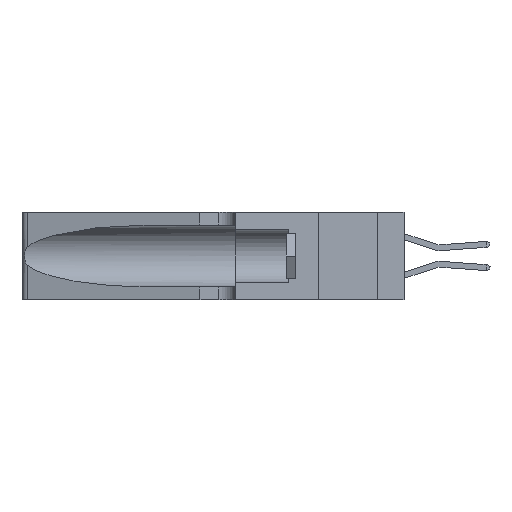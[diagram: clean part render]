
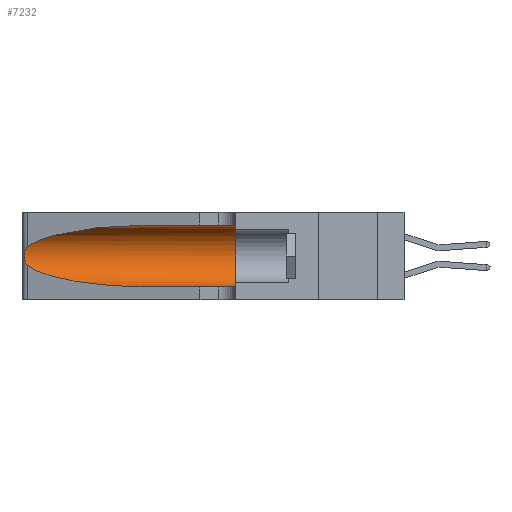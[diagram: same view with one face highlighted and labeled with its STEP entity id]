
A CAD part, left-side view. The second image highlights one B-rep face of the part: STEP entity #7232.
In plain terms, the highlighted cylindrical face has radius 3.308 mm (diameter 6.617 mm), a partial arc.
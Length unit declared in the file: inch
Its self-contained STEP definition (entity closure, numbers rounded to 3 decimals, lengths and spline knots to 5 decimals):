
#592 = FACE_OUTER_BOUND ( 'NONE', #15677, .T. ) ;
#1130 = DIRECTION ( 'NONE',  ( 0., 0., 1. ) ) ;
#1370 = VERTEX_POINT ( 'NONE', #33867 ) ;
#1551 = CARTESIAN_POINT ( 'NONE',  ( 0.25487, 1.22718, 0.14631 ) ) ;
#1865 = EDGE_CURVE ( 'NONE', #4521, #1370, #21527, .T. ) ;
#3967 = CARTESIAN_POINT ( 'NONE',  ( 0.26075, 1.23896, 0.19203 ) ) ;
#4521 = VERTEX_POINT ( 'NONE', #21553 ) ;
#6038 = DIRECTION ( 'NONE',  ( 0., 0., -1. ) ) ;
#6433 = CARTESIAN_POINT ( 'NONE',  ( 0.25487, 1.22718, 0.22369 ) ) ;
#6656 = CARTESIAN_POINT ( 'NONE',  ( 0.25639, 1.23186, 0.15144 ) ) ;
#6766 = CARTESIAN_POINT ( 'NONE',  ( 0.25639, 1.23184, 0.21858 ) ) ;
#7208 = LINE ( 'NONE', #34046, #10570 ) ;
#7232 = ADVANCED_FACE ( 'NONE', ( #592 ), #14036, .F. ) ;
#7325 = ORIENTED_EDGE ( 'NONE', *, *, #1865, .F. ) ;
#9291 = ORIENTED_EDGE ( 'NONE', *, *, #25274, .T. ) ;
#9349 = CARTESIAN_POINT ( 'NONE',  ( 0.25787, 1.23484, 0.2124 ) ) ;
#9441 =( BOUNDED_CURVE ( )  B_SPLINE_CURVE ( 3, ( #29199, #26772, #21514, #10709 ),
 .UNSPECIFIED., .F., .T. ) 
 B_SPLINE_CURVE_WITH_KNOTS ( ( 4, 4 ),
 ( 3.44316, 4.71239 ),
 .UNSPECIFIED. ) 
 CURVE ( )  GEOMETRIC_REPRESENTATION_ITEM ( )  RATIONAL_B_SPLINE_CURVE ( ( 1., 0.87, 0.87, 1. ) ) 
 REPRESENTATION_ITEM ( '' )  );
#10031 = VERTEX_POINT ( 'NONE', #1551 ) ;
#10570 = VECTOR ( 'NONE', #33801, 39.37008 ) ;
#10659 = CARTESIAN_POINT ( 'NONE',  ( 0.1305, 1.61858, 0.31525 ) ) ;
#10709 = CARTESIAN_POINT ( 'NONE',  ( 0.1305, 0.72297, 0.05475 ) ) ;
#11911 = CARTESIAN_POINT ( 'NONE',  ( 0.25555, 1.22993, 0.14849 ) ) ;
#12670 = CARTESIAN_POINT ( 'NONE',  ( 0.18966, 0.96281, 0.31525 ) ) ;
#13134 = DIRECTION ( 'NONE',  ( 0., -1., 0. ) ) ;
#13208 = ORIENTED_EDGE ( 'NONE', *, *, #21748, .T. ) ;
#14036 = CYLINDRICAL_SURFACE ( 'NONE', #29846, 0.13025 ) ;
#14564 = VERTEX_POINT ( 'NONE', #17581 ) ;
#14617 = EDGE_CURVE ( 'NONE', #4521, #14564, #18278, .T. ) ;
#15677 = EDGE_LOOP ( 'NONE', ( #31311, #9291, #13208, #22626, #17065, #7325 ) ) ;
#17065 = ORIENTED_EDGE ( 'NONE', *, *, #29826, .F. ) ;
#17087 = CARTESIAN_POINT ( 'NONE',  ( 0.26075, 1.23896, 0.178 ) ) ;
#17581 = CARTESIAN_POINT ( 'NONE',  ( 0.25487, 1.22718, 0.22369 ) ) ;
#18278 =( BOUNDED_CURVE ( )  B_SPLINE_CURVE ( 3, ( #22957, #12670, #31363, #28329 ),
 .UNSPECIFIED., .F., .T. ) 
 B_SPLINE_CURVE_WITH_KNOTS ( ( 4, 4 ),
 ( 1.5708, 2.84003 ),
 .UNSPECIFIED. ) 
 CURVE ( )  GEOMETRIC_REPRESENTATION_ITEM ( )  RATIONAL_B_SPLINE_CURVE ( ( 1., 0.87, 0.87, 1. ) ) 
 REPRESENTATION_ITEM ( '' )  );
#18868 = CARTESIAN_POINT ( 'NONE',  ( 0.1305, 0.72297, 0.05475 ) ) ;
#18933 = DIRECTION ( 'NONE',  ( 0., -1., 0. ) ) ;
#19793 = CARTESIAN_POINT ( 'NONE',  ( 0.25854, 1.2359, 0.20912 ) ) ;
#20022 = CARTESIAN_POINT ( 'NONE',  ( 0.25555, 1.22994, 0.2215 ) ) ;
#20241 = CARTESIAN_POINT ( 'NONE',  ( 0.1305, 0.35, 0.185 ) ) ;
#21514 = CARTESIAN_POINT ( 'NONE',  ( 0.18966, 0.96281, 0.05475 ) ) ;
#21527 = LINE ( 'NONE', #10659, #31530 ) ;
#21553 = CARTESIAN_POINT ( 'NONE',  ( 0.1305, 0.72297, 0.31525 ) ) ;
#21748 = EDGE_CURVE ( 'NONE', #10031, #32441, #9441, .T. ) ;
#22071 = CARTESIAN_POINT ( 'NONE',  ( 0.1305, 1.61858, 0.185 ) ) ;
#22167 = VERTEX_POINT ( 'NONE', #32015 ) ;
#22487 = CARTESIAN_POINT ( 'NONE',  ( 0.26017, 1.23833, 0.17102 ) ) ;
#22626 = ORIENTED_EDGE ( 'NONE', *, *, #29949, .T. ) ;
#22706 = CARTESIAN_POINT ( 'NONE',  ( 0.25856, 1.23593, 0.16098 ) ) ;
#22957 = CARTESIAN_POINT ( 'NONE',  ( 0.1305, 0.72297, 0.31525 ) ) ;
#25172 = CARTESIAN_POINT ( 'NONE',  ( 0.25487, 1.22718, 0.14631 ) ) ;
#25274 = EDGE_CURVE ( 'NONE', #14564, #10031, #34359, .T. ) ;
#25672 = CIRCLE ( 'NONE', #26285, 0.13025 ) ;
#26285 = AXIS2_PLACEMENT_3D ( 'NONE', #20241, #30379, #1130 ) ;
#26772 = CARTESIAN_POINT ( 'NONE',  ( 0.2373, 1.15595, 0.08982 ) ) ;
#28329 = CARTESIAN_POINT ( 'NONE',  ( 0.25487, 1.22718, 0.22369 ) ) ;
#29199 = CARTESIAN_POINT ( 'NONE',  ( 0.25487, 1.22718, 0.14631 ) ) ;
#29826 = EDGE_CURVE ( 'NONE', #1370, #22167, #25672, .T. ) ;
#29846 = AXIS2_PLACEMENT_3D ( 'NONE', #22071, #18933, #6038 ) ;
#29949 = EDGE_CURVE ( 'NONE', #32441, #22167, #7208, .T. ) ;
#30379 = DIRECTION ( 'NONE',  ( 0., 1., 0. ) ) ;
#30505 = CARTESIAN_POINT ( 'NONE',  ( 0.26018, 1.23835, 0.19895 ) ) ;
#31311 = ORIENTED_EDGE ( 'NONE', *, *, #14617, .T. ) ;
#31363 = CARTESIAN_POINT ( 'NONE',  ( 0.2373, 1.15595, 0.28018 ) ) ;
#31530 = VECTOR ( 'NONE', #13134, 39.37008 ) ;
#32015 = CARTESIAN_POINT ( 'NONE',  ( 0.1305, 0.35, 0.05475 ) ) ;
#32441 = VERTEX_POINT ( 'NONE', #18868 ) ;
#33232 = CARTESIAN_POINT ( 'NONE',  ( 0.25789, 1.23486, 0.15765 ) ) ;
#33801 = DIRECTION ( 'NONE',  ( 0., -1., 0. ) ) ;
#33867 = CARTESIAN_POINT ( 'NONE',  ( 0.1305, 0.35, 0.31525 ) ) ;
#34046 = CARTESIAN_POINT ( 'NONE',  ( 0.1305, 1.61858, 0.05475 ) ) ;
#34359 = B_SPLINE_CURVE_WITH_KNOTS ( 'NONE', 3,
 ( #6433, #20022, #6766, #9349, #19793, #30505, #3967, #17087, #22487, #22706, #33232, #6656, #11911, #25172 ),
 .UNSPECIFIED., .F., .F.,
 ( 4, 2, 2, 2, 2, 2, 4 ),
 ( 0., 0.00027, 0.00053, 0.00107, 0.0016, 0.00187, 0.00214 ),
 .UNSPECIFIED. ) ;
